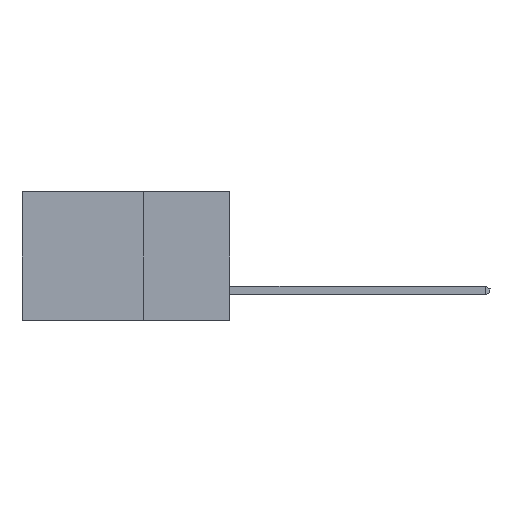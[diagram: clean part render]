
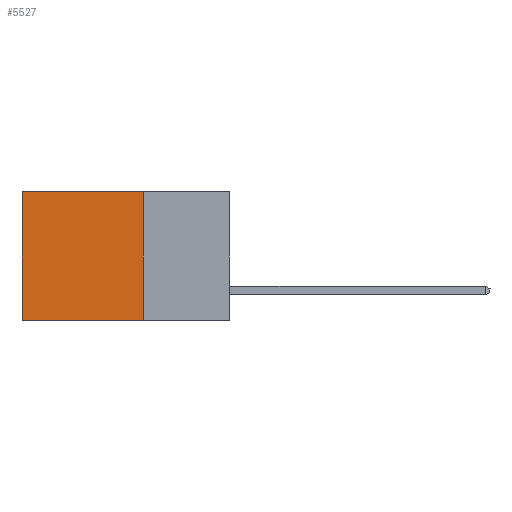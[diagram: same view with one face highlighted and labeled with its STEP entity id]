
A CAD part, left-side view. The second image highlights one B-rep face of the part: STEP entity #5527.
In plain terms, the highlighted planar face has unit normal (-1, 0, 0).
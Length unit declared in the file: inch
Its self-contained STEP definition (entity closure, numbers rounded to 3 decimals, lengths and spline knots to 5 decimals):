
#186 = LINE ( 'NONE', #8581, #3499 ) ;
#288 = FACE_OUTER_BOUND ( 'NONE', #15981, .T. ) ;
#1238 = CARTESIAN_POINT ( 'NONE',  ( 0.2615, 0.25, -0.37 ) ) ;
#1386 = CARTESIAN_POINT ( 'NONE',  ( 0.2615, 0.25, -0.37 ) ) ;
#1865 = VERTEX_POINT ( 'NONE', #10797 ) ;
#3145 = EDGE_CURVE ( 'NONE', #14141, #1865, #4436, .T. ) ;
#3499 = VECTOR ( 'NONE', #7197, 39.37008 ) ;
#3800 = DIRECTION ( 'NONE',  ( 0., 1., 0. ) ) ;
#4166 = VECTOR ( 'NONE', #15997, 39.37008 ) ;
#4436 = LINE ( 'NONE', #12559, #4166 ) ;
#4616 = ORIENTED_EDGE ( 'NONE', *, *, #13307, .F. ) ;
#5520 = LINE ( 'NONE', #9628, #11724 ) ;
#5527 = ADVANCED_FACE ( 'NONE', ( #288 ), #7306, .F. ) ;
#6726 = ORIENTED_EDGE ( 'NONE', *, *, #3145, .T. ) ;
#7197 = DIRECTION ( 'NONE',  ( 0., 1., 0. ) ) ;
#7306 = PLANE ( 'NONE',  #14249 ) ;
#7906 = EDGE_CURVE ( 'NONE', #13985, #14141, #13654, .T. ) ;
#8076 = DIRECTION ( 'NONE',  ( 0., 0., -1. ) ) ;
#8581 = CARTESIAN_POINT ( 'NONE',  ( 0.2615, 0.25, -0.37 ) ) ;
#9476 = ORIENTED_EDGE ( 'NONE', *, *, #10502, .F. ) ;
#9628 = CARTESIAN_POINT ( 'NONE',  ( 0.2615, 0.25, -0.37 ) ) ;
#10502 = EDGE_CURVE ( 'NONE', #14687, #1865, #186, .T. ) ;
#10662 = CARTESIAN_POINT ( 'NONE',  ( 0.2615, 0.25, 0. ) ) ;
#10797 = CARTESIAN_POINT ( 'NONE',  ( 0.2615, 0.6, -0.37 ) ) ;
#11336 = DIRECTION ( 'NONE',  ( 1., 0., 0. ) ) ;
#11724 = VECTOR ( 'NONE', #8076, 39.37008 ) ;
#12559 = CARTESIAN_POINT ( 'NONE',  ( 0.2615, 0.6, -0.37 ) ) ;
#13303 = CARTESIAN_POINT ( 'NONE',  ( 0.2615, 0.6, 0. ) ) ;
#13307 = EDGE_CURVE ( 'NONE', #13985, #14687, #5520, .T. ) ;
#13594 = VECTOR ( 'NONE', #3800, 39.37008 ) ;
#13654 = LINE ( 'NONE', #17494, #13594 ) ;
#13985 = VERTEX_POINT ( 'NONE', #10662 ) ;
#14141 = VERTEX_POINT ( 'NONE', #13303 ) ;
#14249 = AXIS2_PLACEMENT_3D ( 'NONE', #1386, #11336, #16894 ) ;
#14687 = VERTEX_POINT ( 'NONE', #1238 ) ;
#15217 = ORIENTED_EDGE ( 'NONE', *, *, #7906, .T. ) ;
#15981 = EDGE_LOOP ( 'NONE', ( #6726, #9476, #4616, #15217 ) ) ;
#15997 = DIRECTION ( 'NONE',  ( 0., 0., -1. ) ) ;
#16894 = DIRECTION ( 'NONE',  ( 0., 0., -1. ) ) ;
#17494 = CARTESIAN_POINT ( 'NONE',  ( 0.2615, 0.25, 0. ) ) ;
